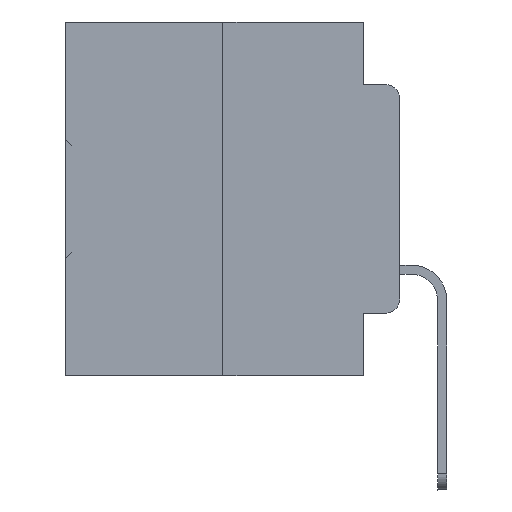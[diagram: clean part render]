
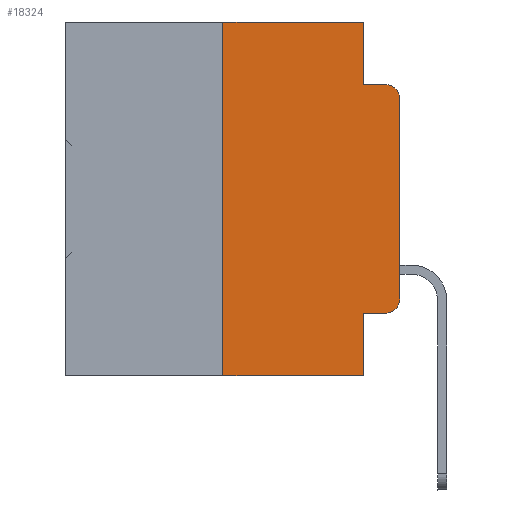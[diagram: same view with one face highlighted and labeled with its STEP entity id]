
A CAD part, left-side view. The second image highlights one B-rep face of the part: STEP entity #18324.
In plain terms, the highlighted planar face has unit normal (-1, 0, 0).
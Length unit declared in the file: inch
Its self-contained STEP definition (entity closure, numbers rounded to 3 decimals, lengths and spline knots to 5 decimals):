
#123 = VECTOR ( 'NONE', #27399, 39.37008 ) ;
#558 = VERTEX_POINT ( 'NONE', #36490 ) ;
#965 = LINE ( 'NONE', #17970, #4485 ) ;
#1521 = CARTESIAN_POINT ( 'NONE',  ( 0., 0.051, -0.4115 ) ) ;
#1963 = VERTEX_POINT ( 'NONE', #5298 ) ;
#2082 = VECTOR ( 'NONE', #10086, 39.37008 ) ;
#2990 = DIRECTION ( 'NONE',  ( 0., 0., 1. ) ) ;
#3049 = CARTESIAN_POINT ( 'NONE',  ( 0., 0.02, -0.3915 ) ) ;
#3640 = AXIS2_PLACEMENT_3D ( 'NONE', #5648, #16919, #22641 ) ;
#3687 = DIRECTION ( 'NONE',  ( 0., 0., -1. ) ) ;
#4182 = ORIENTED_EDGE ( 'NONE', *, *, #36154, .T. ) ;
#4461 = VECTOR ( 'NONE', #3687, 39.37008 ) ;
#4485 = VECTOR ( 'NONE', #14479, 39.37008 ) ;
#5083 = EDGE_LOOP ( 'NONE', ( #4182, #11977, #17536, #35122, #26868, #35380, #35274, #14657, #17705, #10728 ) ) ;
#5298 = CARTESIAN_POINT ( 'NONE',  ( 0., 0.25, 0. ) ) ;
#5426 = LINE ( 'NONE', #14796, #4461 ) ;
#5648 = CARTESIAN_POINT ( 'NONE',  ( 0., 0.473, 0. ) ) ;
#6527 = CIRCLE ( 'NONE', #7123, 0.02 ) ;
#7123 = AXIS2_PLACEMENT_3D ( 'NONE', #3049, #34295, #34105 ) ;
#7813 = CARTESIAN_POINT ( 'NONE',  ( 0., 0.473, 0. ) ) ;
#8146 = CARTESIAN_POINT ( 'NONE',  ( 0., 0.02, -0.4115 ) ) ;
#8654 = DIRECTION ( 'NONE',  ( 0., -1., 0. ) ) ;
#9837 = CARTESIAN_POINT ( 'NONE',  ( 0., 0.051, 0. ) ) ;
#10086 = DIRECTION ( 'NONE',  ( 0., 0., -1. ) ) ;
#10264 = CARTESIAN_POINT ( 'NONE',  ( 0., 0.051, 0. ) ) ;
#10373 = VECTOR ( 'NONE', #36130, 39.37008 ) ;
#10728 = ORIENTED_EDGE ( 'NONE', *, *, #17121, .T. ) ;
#11010 = DIRECTION ( 'NONE',  ( -1., 0., 0. ) ) ;
#11230 = EDGE_CURVE ( 'NONE', #27854, #34795, #17900, .T. ) ;
#11683 = VECTOR ( 'NONE', #8654, 39.37008 ) ;
#11977 = ORIENTED_EDGE ( 'NONE', *, *, #34334, .T. ) ;
#13032 = LINE ( 'NONE', #10264, #2082 ) ;
#13391 = LINE ( 'NONE', #13582, #10373 ) ;
#13582 = CARTESIAN_POINT ( 'NONE',  ( 0., 0.473, -0.5 ) ) ;
#13660 = VECTOR ( 'NONE', #29177, 39.37008 ) ;
#14479 = DIRECTION ( 'NONE',  ( 0., 0., 1. ) ) ;
#14640 = CARTESIAN_POINT ( 'NONE',  ( 0., 0., 0. ) ) ;
#14657 = ORIENTED_EDGE ( 'NONE', *, *, #23169, .F. ) ;
#14796 = CARTESIAN_POINT ( 'NONE',  ( 0., 0.051, 0. ) ) ;
#14967 = EDGE_CURVE ( 'NONE', #21022, #28459, #23423, .T. ) ;
#15059 = CARTESIAN_POINT ( 'NONE',  ( 0., 0., -0.1085 ) ) ;
#16919 = DIRECTION ( 'NONE',  ( 1., 0., 0. ) ) ;
#17121 = EDGE_CURVE ( 'NONE', #34795, #30101, #6527, .T. ) ;
#17536 = ORIENTED_EDGE ( 'NONE', *, *, #14967, .F. ) ;
#17705 = ORIENTED_EDGE ( 'NONE', *, *, #11230, .T. ) ;
#17900 = LINE ( 'NONE', #18452, #13660 ) ;
#17970 = CARTESIAN_POINT ( 'NONE',  ( 0., 0.25, 0. ) ) ;
#18324 = ADVANCED_FACE ( 'NONE', ( #19695 ), #30970, .F. ) ;
#18452 = CARTESIAN_POINT ( 'NONE',  ( 0., 0.051, -0.4115 ) ) ;
#19064 = EDGE_CURVE ( 'NONE', #1963, #20251, #33675, .T. ) ;
#19675 = DIRECTION ( 'NONE',  ( 0., 0., -1. ) ) ;
#19695 = FACE_OUTER_BOUND ( 'NONE', #5083, .T. ) ;
#19754 = CARTESIAN_POINT ( 'NONE',  ( 0., 0., -0.3915 ) ) ;
#19980 = CARTESIAN_POINT ( 'NONE',  ( 0., 0.02, -0.0885 ) ) ;
#20251 = VERTEX_POINT ( 'NONE', #9837 ) ;
#21022 = VERTEX_POINT ( 'NONE', #29831 ) ;
#21382 = CARTESIAN_POINT ( 'NONE',  ( 0., 0.25, -0.5 ) ) ;
#22534 = VERTEX_POINT ( 'NONE', #21382 ) ;
#22641 = DIRECTION ( 'NONE',  ( 0., 0., -1. ) ) ;
#22948 = EDGE_CURVE ( 'NONE', #20251, #21022, #13032, .T. ) ;
#22998 = EDGE_CURVE ( 'NONE', #22534, #558, #13391, .T. ) ;
#23169 = EDGE_CURVE ( 'NONE', #27854, #558, #5426, .T. ) ;
#23423 = LINE ( 'NONE', #34714, #11683 ) ;
#24104 = VERTEX_POINT ( 'NONE', #15059 ) ;
#26868 = ORIENTED_EDGE ( 'NONE', *, *, #19064, .F. ) ;
#27399 = DIRECTION ( 'NONE',  ( 0., -1., 0. ) ) ;
#27655 = EDGE_CURVE ( 'NONE', #22534, #1963, #965, .T. ) ;
#27854 = VERTEX_POINT ( 'NONE', #1521 ) ;
#28204 = CIRCLE ( 'NONE', #32358, 0.02 ) ;
#28459 = VERTEX_POINT ( 'NONE', #19980 ) ;
#29177 = DIRECTION ( 'NONE',  ( 0., -1., 0. ) ) ;
#29831 = CARTESIAN_POINT ( 'NONE',  ( 0., 0.051, -0.0885 ) ) ;
#30101 = VERTEX_POINT ( 'NONE', #19754 ) ;
#30970 = PLANE ( 'NONE',  #3640 ) ;
#31827 = LINE ( 'NONE', #14640, #33045 ) ;
#32358 = AXIS2_PLACEMENT_3D ( 'NONE', #33733, #11010, #19675 ) ;
#33045 = VECTOR ( 'NONE', #2990, 39.37008 ) ;
#33675 = LINE ( 'NONE', #7813, #123 ) ;
#33733 = CARTESIAN_POINT ( 'NONE',  ( 0., 0.02, -0.1085 ) ) ;
#34105 = DIRECTION ( 'NONE',  ( 0., 0., -1. ) ) ;
#34295 = DIRECTION ( 'NONE',  ( -1., 0., 0. ) ) ;
#34334 = EDGE_CURVE ( 'NONE', #24104, #28459, #28204, .T. ) ;
#34714 = CARTESIAN_POINT ( 'NONE',  ( 0., 0.051, -0.0885 ) ) ;
#34795 = VERTEX_POINT ( 'NONE', #8146 ) ;
#35122 = ORIENTED_EDGE ( 'NONE', *, *, #22948, .F. ) ;
#35274 = ORIENTED_EDGE ( 'NONE', *, *, #22998, .T. ) ;
#35380 = ORIENTED_EDGE ( 'NONE', *, *, #27655, .F. ) ;
#36130 = DIRECTION ( 'NONE',  ( 0., -1., 0. ) ) ;
#36154 = EDGE_CURVE ( 'NONE', #30101, #24104, #31827, .T. ) ;
#36490 = CARTESIAN_POINT ( 'NONE',  ( 0., 0.051, -0.5 ) ) ;
